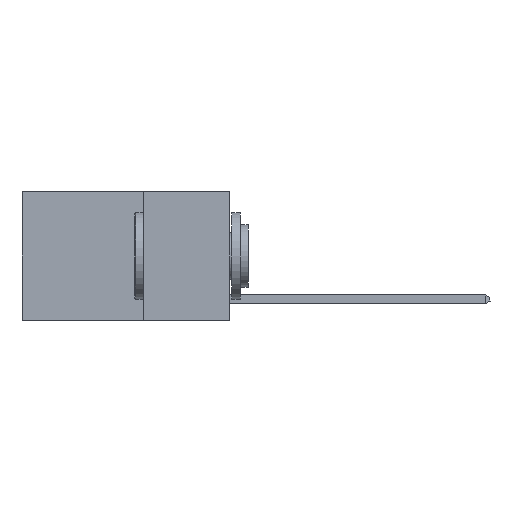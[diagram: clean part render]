
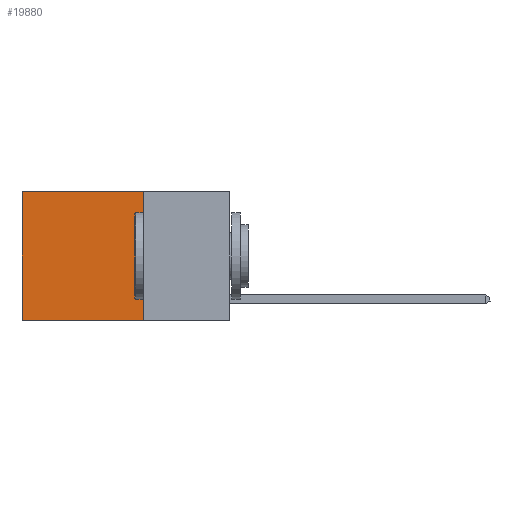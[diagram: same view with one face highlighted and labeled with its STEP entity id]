
A CAD part, left-side view. The second image highlights one B-rep face of the part: STEP entity #19880.
In plain terms, the highlighted planar face has unit normal (-1, 0, 0).
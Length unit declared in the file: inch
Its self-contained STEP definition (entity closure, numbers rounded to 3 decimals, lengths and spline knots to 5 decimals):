
#2041 = DIRECTION ( 'NONE',  ( 0., 1., 0. ) ) ;
#2622 = CARTESIAN_POINT ( 'NONE',  ( 0.2625, 0.25, 0. ) ) ;
#3920 = CARTESIAN_POINT ( 'NONE',  ( 0.2625, 0.25, 0. ) ) ;
#4461 = AXIS2_PLACEMENT_3D ( 'NONE', #2622, #15281, #7090 ) ;
#5958 = LINE ( 'NONE', #10849, #10122 ) ;
#6349 = VERTEX_POINT ( 'NONE', #7922 ) ;
#6428 = VERTEX_POINT ( 'NONE', #10411 ) ;
#6593 = VECTOR ( 'NONE', #2041, 39.37008 ) ;
#6986 = EDGE_CURVE ( 'NONE', #8246, #6349, #13160, .T. ) ;
#7090 = DIRECTION ( 'NONE',  ( 0., 0., -1. ) ) ;
#7229 = ORIENTED_EDGE ( 'NONE', *, *, #6986, .T. ) ;
#7308 = ORIENTED_EDGE ( 'NONE', *, *, #19523, .F. ) ;
#7809 = ORIENTED_EDGE ( 'NONE', *, *, #12183, .F. ) ;
#7922 = CARTESIAN_POINT ( 'NONE',  ( 0.2625, 0.6, -0.37 ) ) ;
#8059 = VECTOR ( 'NONE', #12013, 39.37008 ) ;
#8246 = VERTEX_POINT ( 'NONE', #8868 ) ;
#8728 = FACE_OUTER_BOUND ( 'NONE', #18351, .T. ) ;
#8868 = CARTESIAN_POINT ( 'NONE',  ( 0.2625, 0.6, 0. ) ) ;
#8969 = VERTEX_POINT ( 'NONE', #9625 ) ;
#9541 = DIRECTION ( 'NONE',  ( 0., 0., -1. ) ) ;
#9625 = CARTESIAN_POINT ( 'NONE',  ( 0.2625, 0.25, 0. ) ) ;
#10122 = VECTOR ( 'NONE', #13938, 39.37008 ) ;
#10411 = CARTESIAN_POINT ( 'NONE',  ( 0.2625, 0.25, -0.37 ) ) ;
#10849 = CARTESIAN_POINT ( 'NONE',  ( 0.2625, 0.25, -0.37 ) ) ;
#12013 = DIRECTION ( 'NONE',  ( 0., 0., -1. ) ) ;
#12083 = PLANE ( 'NONE',  #4461 ) ;
#12183 = EDGE_CURVE ( 'NONE', #6428, #6349, #5958, .T. ) ;
#13160 = LINE ( 'NONE', #17935, #8059 ) ;
#13938 = DIRECTION ( 'NONE',  ( 0., 1., 0. ) ) ;
#13951 = VECTOR ( 'NONE', #9541, 39.37008 ) ;
#14615 = EDGE_CURVE ( 'NONE', #8969, #8246, #16380, .T. ) ;
#15281 = DIRECTION ( 'NONE',  ( 1., 0., 0. ) ) ;
#16380 = LINE ( 'NONE', #3920, #6593 ) ;
#17547 = ORIENTED_EDGE ( 'NONE', *, *, #14615, .T. ) ;
#17935 = CARTESIAN_POINT ( 'NONE',  ( 0.2625, 0.6, 0. ) ) ;
#18351 = EDGE_LOOP ( 'NONE', ( #7229, #7809, #7308, #17547 ) ) ;
#18823 = CARTESIAN_POINT ( 'NONE',  ( 0.2625, 0.25, 0. ) ) ;
#19523 = EDGE_CURVE ( 'NONE', #8969, #6428, #20356, .T. ) ;
#19880 = ADVANCED_FACE ( 'NONE', ( #8728 ), #12083, .F. ) ;
#20356 = LINE ( 'NONE', #18823, #13951 ) ;
